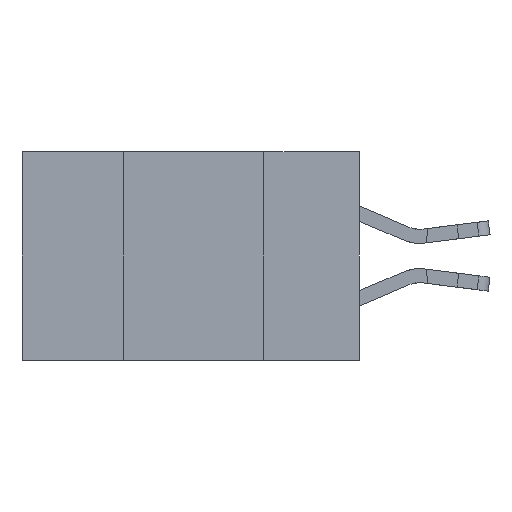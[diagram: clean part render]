
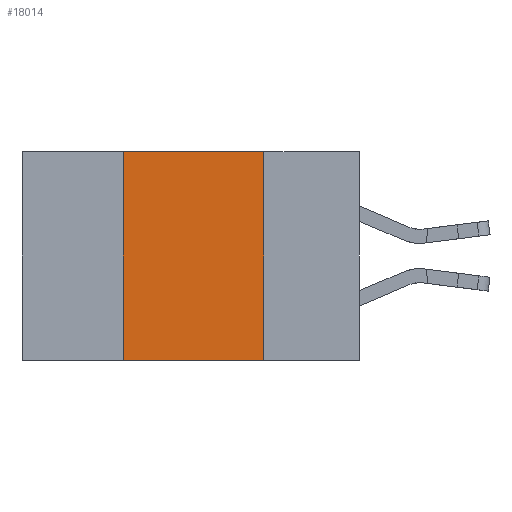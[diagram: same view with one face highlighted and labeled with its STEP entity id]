
A CAD part, left-side view. The second image highlights one B-rep face of the part: STEP entity #18014.
In plain terms, the highlighted planar face has unit normal (-1, 0, 0).
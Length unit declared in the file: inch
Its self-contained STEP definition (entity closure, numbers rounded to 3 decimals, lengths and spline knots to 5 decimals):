
#428 = DIRECTION ( 'NONE',  ( 0., 0., 1. ) ) ;
#636 = LINE ( 'NONE', #19648, #7162 ) ;
#885 = FACE_OUTER_BOUND ( 'NONE', #3645, .T. ) ;
#1301 = PLANE ( 'NONE',  #5795 ) ;
#1521 = DIRECTION ( 'NONE',  ( 1., 0., 0. ) ) ;
#1879 = CARTESIAN_POINT ( 'NONE',  ( 0., 0.6, -0.37 ) ) ;
#2686 = EDGE_CURVE ( 'NONE', #7370, #14866, #13071, .T. ) ;
#2989 = CARTESIAN_POINT ( 'NONE',  ( 0., 0.6, 0. ) ) ;
#3410 = LINE ( 'NONE', #17067, #19653 ) ;
#3645 = EDGE_LOOP ( 'NONE', ( #13354, #21319, #4369, #19842 ) ) ;
#4369 = ORIENTED_EDGE ( 'NONE', *, *, #11463, .F. ) ;
#4573 = EDGE_CURVE ( 'NONE', #9808, #18320, #14548, .T. ) ;
#5795 = AXIS2_PLACEMENT_3D ( 'NONE', #2989, #1521, #8437 ) ;
#6382 = EDGE_CURVE ( 'NONE', #18320, #14866, #636, .T. ) ;
#6562 = CARTESIAN_POINT ( 'NONE',  ( 0., 0.42, 0. ) ) ;
#7162 = VECTOR ( 'NONE', #9614, 39.37008 ) ;
#7370 = VERTEX_POINT ( 'NONE', #20770 ) ;
#7855 = CARTESIAN_POINT ( 'NONE',  ( 0., 0.17, 0. ) ) ;
#8437 = DIRECTION ( 'NONE',  ( 0., 0., -1. ) ) ;
#9614 = DIRECTION ( 'NONE',  ( 0., 0., -1. ) ) ;
#9658 = VECTOR ( 'NONE', #13571, 39.37008 ) ;
#9808 = VERTEX_POINT ( 'NONE', #6562 ) ;
#11463 = EDGE_CURVE ( 'NONE', #7370, #9808, #3410, .T. ) ;
#13071 = LINE ( 'NONE', #1879, #9658 ) ;
#13354 = ORIENTED_EDGE ( 'NONE', *, *, #6382, .F. ) ;
#13571 = DIRECTION ( 'NONE',  ( 0., -1., 0. ) ) ;
#14548 = LINE ( 'NONE', #21526, #18491 ) ;
#14866 = VERTEX_POINT ( 'NONE', #17011 ) ;
#17011 = CARTESIAN_POINT ( 'NONE',  ( 0., 0.17, -0.37 ) ) ;
#17067 = CARTESIAN_POINT ( 'NONE',  ( 0., 0.42, 0. ) ) ;
#18014 = ADVANCED_FACE ( 'NONE', ( #885 ), #1301, .F. ) ;
#18036 = DIRECTION ( 'NONE',  ( 0., -1., 0. ) ) ;
#18320 = VERTEX_POINT ( 'NONE', #7855 ) ;
#18491 = VECTOR ( 'NONE', #18036, 39.37008 ) ;
#19648 = CARTESIAN_POINT ( 'NONE',  ( 0., 0.17, 0. ) ) ;
#19653 = VECTOR ( 'NONE', #428, 39.37008 ) ;
#19842 = ORIENTED_EDGE ( 'NONE', *, *, #2686, .T. ) ;
#20770 = CARTESIAN_POINT ( 'NONE',  ( 0., 0.42, -0.37 ) ) ;
#21319 = ORIENTED_EDGE ( 'NONE', *, *, #4573, .F. ) ;
#21526 = CARTESIAN_POINT ( 'NONE',  ( 0., 0.6, 0. ) ) ;
